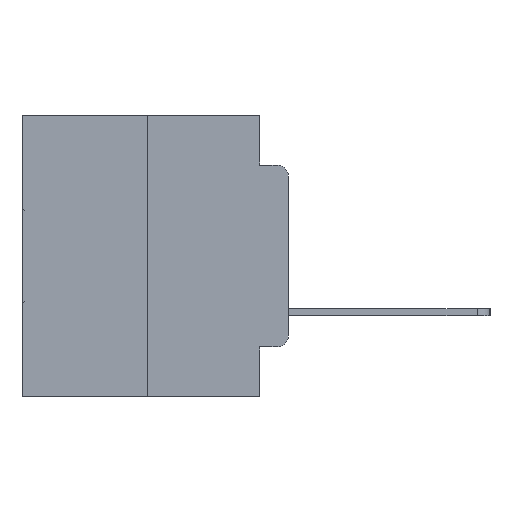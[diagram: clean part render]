
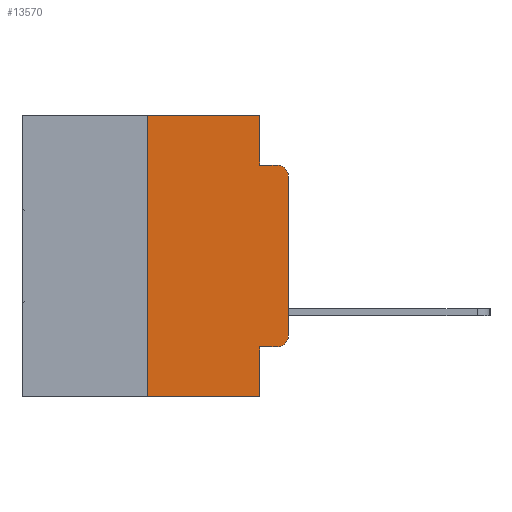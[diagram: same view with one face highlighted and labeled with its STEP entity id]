
A CAD part, left-side view. The second image highlights one B-rep face of the part: STEP entity #13570.
In plain terms, the highlighted planar face has unit normal (-1, 0, 0).
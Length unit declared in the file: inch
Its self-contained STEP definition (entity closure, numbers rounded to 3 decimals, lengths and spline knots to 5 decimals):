
#495 = EDGE_CURVE ( 'NONE', #12414, #27162, #4594, .T. ) ;
#536 = DIRECTION ( 'NONE',  ( 0., 0., -1. ) ) ;
#1065 = DIRECTION ( 'NONE',  ( 0., 0., -1. ) ) ;
#1615 = VERTEX_POINT ( 'NONE', #3663 ) ;
#2231 = LINE ( 'NONE', #27756, #3703 ) ;
#2589 = VERTEX_POINT ( 'NONE', #17135 ) ;
#3075 = CIRCLE ( 'NONE', #15670, 0.02 ) ;
#3179 = ORIENTED_EDGE ( 'NONE', *, *, #29129, .T. ) ;
#3280 = EDGE_CURVE ( 'NONE', #12414, #6024, #11826, .T. ) ;
#3663 = CARTESIAN_POINT ( 'NONE',  ( 0., 0.051, -0.0885 ) ) ;
#3703 = VECTOR ( 'NONE', #14316, 39.37008 ) ;
#4594 = LINE ( 'NONE', #17368, #10081 ) ;
#4931 = DIRECTION ( 'NONE',  ( -1., 0., 0. ) ) ;
#5356 = CARTESIAN_POINT ( 'NONE',  ( 0., 0.051, 0. ) ) ;
#5623 = EDGE_CURVE ( 'NONE', #2589, #12269, #16638, .T. ) ;
#5994 = CARTESIAN_POINT ( 'NONE',  ( 0., 0.25, 0. ) ) ;
#6024 = VERTEX_POINT ( 'NONE', #11880 ) ;
#7164 = EDGE_LOOP ( 'NONE', ( #21073, #26988, #16479, #17211, #18633, #24579, #13984, #25949, #14722, #3179 ) ) ;
#7470 = LINE ( 'NONE', #25664, #18930 ) ;
#8195 = CARTESIAN_POINT ( 'NONE',  ( 0., 0.473, 0. ) ) ;
#8382 = DIRECTION ( 'NONE',  ( 0., 0., 1. ) ) ;
#9524 = VECTOR ( 'NONE', #21283, 39.37008 ) ;
#9650 = AXIS2_PLACEMENT_3D ( 'NONE', #18707, #4931, #20960 ) ;
#10081 = VECTOR ( 'NONE', #24942, 39.37008 ) ;
#10112 = CARTESIAN_POINT ( 'NONE',  ( 0., 0.25, -0.5 ) ) ;
#10556 = VERTEX_POINT ( 'NONE', #10112 ) ;
#11398 = CARTESIAN_POINT ( 'NONE',  ( 0., 0.02, -0.0885 ) ) ;
#11826 = LINE ( 'NONE', #5356, #16431 ) ;
#11880 = CARTESIAN_POINT ( 'NONE',  ( 0., 0.051, -0.5 ) ) ;
#12213 = DIRECTION ( 'NONE',  ( 0., 0., -1. ) ) ;
#12269 = VERTEX_POINT ( 'NONE', #20764 ) ;
#12414 = VERTEX_POINT ( 'NONE', #21639 ) ;
#12436 = AXIS2_PLACEMENT_3D ( 'NONE', #27870, #14430, #536 ) ;
#13570 = ADVANCED_FACE ( 'NONE', ( #14286 ), #25536, .F. ) ;
#13816 = DIRECTION ( 'NONE',  ( 0., 0., -1. ) ) ;
#13984 = ORIENTED_EDGE ( 'NONE', *, *, #21220, .T. ) ;
#14131 = VERTEX_POINT ( 'NONE', #11398 ) ;
#14225 = EDGE_CURVE ( 'NONE', #12269, #1615, #7470, .T. ) ;
#14286 = FACE_OUTER_BOUND ( 'NONE', #7164, .T. ) ;
#14316 = DIRECTION ( 'NONE',  ( 0., -1., 0. ) ) ;
#14332 = VERTEX_POINT ( 'NONE', #28282 ) ;
#14430 = DIRECTION ( 'NONE',  ( 1., 0., 0. ) ) ;
#14722 = ORIENTED_EDGE ( 'NONE', *, *, #495, .T. ) ;
#14930 = DIRECTION ( 'NONE',  ( -1., 0., 0. ) ) ;
#14972 = EDGE_CURVE ( 'NONE', #14332, #14131, #3075, .T. ) ;
#15670 = AXIS2_PLACEMENT_3D ( 'NONE', #28340, #14930, #1065 ) ;
#15915 = VECTOR ( 'NONE', #26253, 39.37008 ) ;
#16431 = VECTOR ( 'NONE', #13816, 39.37008 ) ;
#16479 = ORIENTED_EDGE ( 'NONE', *, *, #17123, .F. ) ;
#16638 = LINE ( 'NONE', #8195, #15915 ) ;
#17123 = EDGE_CURVE ( 'NONE', #1615, #14131, #21611, .T. ) ;
#17135 = CARTESIAN_POINT ( 'NONE',  ( 0., 0.25, 0. ) ) ;
#17211 = ORIENTED_EDGE ( 'NONE', *, *, #14225, .F. ) ;
#17368 = CARTESIAN_POINT ( 'NONE',  ( 0., 0.051, -0.4115 ) ) ;
#18116 = EDGE_CURVE ( 'NONE', #25905, #14332, #25353, .T. ) ;
#18157 = VECTOR ( 'NONE', #8382, 39.37008 ) ;
#18633 = ORIENTED_EDGE ( 'NONE', *, *, #5623, .F. ) ;
#18707 = CARTESIAN_POINT ( 'NONE',  ( 0., 0.02, -0.3915 ) ) ;
#18930 = VECTOR ( 'NONE', #12213, 39.37008 ) ;
#19131 = CARTESIAN_POINT ( 'NONE',  ( 0., 0.051, -0.0885 ) ) ;
#19566 = CARTESIAN_POINT ( 'NONE',  ( 0., 0.02, -0.4115 ) ) ;
#20764 = CARTESIAN_POINT ( 'NONE',  ( 0., 0.051, 0. ) ) ;
#20960 = DIRECTION ( 'NONE',  ( 0., 0., -1. ) ) ;
#21073 = ORIENTED_EDGE ( 'NONE', *, *, #18116, .T. ) ;
#21220 = EDGE_CURVE ( 'NONE', #10556, #6024, #2231, .T. ) ;
#21283 = DIRECTION ( 'NONE',  ( 0., -1., 0. ) ) ;
#21611 = LINE ( 'NONE', #19131, #9524 ) ;
#21639 = CARTESIAN_POINT ( 'NONE',  ( 0., 0.051, -0.4115 ) ) ;
#21654 = CIRCLE ( 'NONE', #9650, 0.02 ) ;
#24579 = ORIENTED_EDGE ( 'NONE', *, *, #25459, .F. ) ;
#24681 = VECTOR ( 'NONE', #29185, 39.37008 ) ;
#24726 = CARTESIAN_POINT ( 'NONE',  ( 0., 0., 0. ) ) ;
#24942 = DIRECTION ( 'NONE',  ( 0., -1., 0. ) ) ;
#25353 = LINE ( 'NONE', #24726, #24681 ) ;
#25459 = EDGE_CURVE ( 'NONE', #10556, #2589, #25481, .T. ) ;
#25481 = LINE ( 'NONE', #5994, #18157 ) ;
#25536 = PLANE ( 'NONE',  #12436 ) ;
#25664 = CARTESIAN_POINT ( 'NONE',  ( 0., 0.051, 0. ) ) ;
#25807 = CARTESIAN_POINT ( 'NONE',  ( 0., 0., -0.3915 ) ) ;
#25905 = VERTEX_POINT ( 'NONE', #25807 ) ;
#25949 = ORIENTED_EDGE ( 'NONE', *, *, #3280, .F. ) ;
#26253 = DIRECTION ( 'NONE',  ( 0., -1., 0. ) ) ;
#26988 = ORIENTED_EDGE ( 'NONE', *, *, #14972, .T. ) ;
#27162 = VERTEX_POINT ( 'NONE', #19566 ) ;
#27756 = CARTESIAN_POINT ( 'NONE',  ( 0., 0.473, -0.5 ) ) ;
#27870 = CARTESIAN_POINT ( 'NONE',  ( 0., 0.473, 0. ) ) ;
#28282 = CARTESIAN_POINT ( 'NONE',  ( 0., 0., -0.1085 ) ) ;
#28340 = CARTESIAN_POINT ( 'NONE',  ( 0., 0.02, -0.1085 ) ) ;
#29129 = EDGE_CURVE ( 'NONE', #27162, #25905, #21654, .T. ) ;
#29185 = DIRECTION ( 'NONE',  ( 0., 0., 1. ) ) ;
